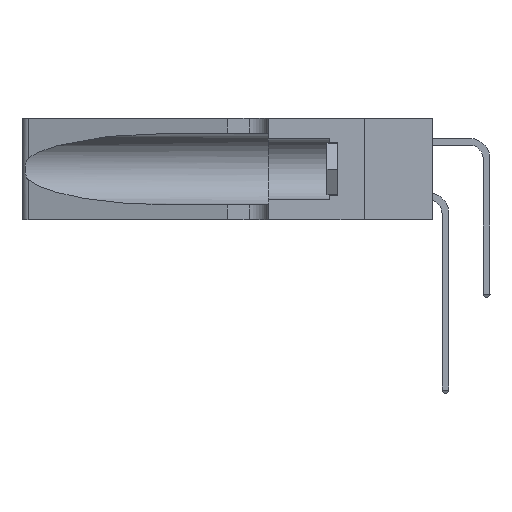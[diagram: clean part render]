
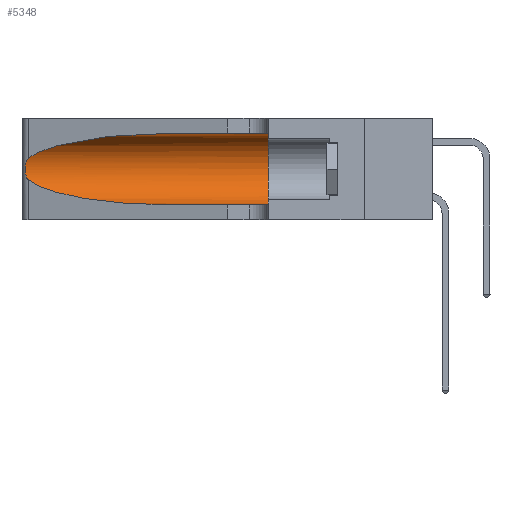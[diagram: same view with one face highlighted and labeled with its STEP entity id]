
A CAD part, left-side view. The second image highlights one B-rep face of the part: STEP entity #5348.
In plain terms, the highlighted cylindrical face has radius 3.308 mm (diameter 6.617 mm), a partial arc.
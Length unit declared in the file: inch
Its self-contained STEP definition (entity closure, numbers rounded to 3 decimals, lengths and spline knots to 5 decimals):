
#450 = B_SPLINE_CURVE_WITH_KNOTS ( 'NONE', 3,
 ( #13901, #22135, #18074, #5650, #20141, #7745, #22219, #9846, #24278, #11929, #26351, #13994, #1385, #16044 ),
 .UNSPECIFIED., .F., .F.,
 ( 4, 2, 2, 2, 2, 2, 4 ),
 ( 0., 0.00027, 0.00053, 0.00107, 0.0016, 0.00187, 0.00214 ),
 .UNSPECIFIED. ) ;
#459 = ORIENTED_EDGE ( 'NONE', *, *, #3956, .T. ) ;
#1385 = CARTESIAN_POINT ( 'NONE',  ( 0.25555, 1.22993, 0.14849 ) ) ;
#1475 =( BOUNDED_CURVE ( )  B_SPLINE_CURVE ( 3, ( #21719, #19643, #15539, #3058 ),
 .UNSPECIFIED., .F., .F. ) 
 B_SPLINE_CURVE_WITH_KNOTS ( ( 4, 4 ),
 ( 3.44316, 4.71239 ),
 .UNSPECIFIED. ) 
 CURVE ( )  GEOMETRIC_REPRESENTATION_ITEM ( )  RATIONAL_B_SPLINE_CURVE ( ( 1., 0.87, 0.87, 1. ) ) 
 REPRESENTATION_ITEM ( '' )  );
#1783 = LINE ( 'NONE', #19438, #17848 ) ;
#1936 = FACE_OUTER_BOUND ( 'NONE', #20420, .T. ) ;
#2734 = CARTESIAN_POINT ( 'NONE',  ( 0.1305, 0.35, 0.05475 ) ) ;
#3058 = CARTESIAN_POINT ( 'NONE',  ( 0.1305, 0.72297, 0.05475 ) ) ;
#3063 = VERTEX_POINT ( 'NONE', #4039 ) ;
#3956 = EDGE_CURVE ( 'NONE', #25879, #3063, #1475, .T. ) ;
#4039 = CARTESIAN_POINT ( 'NONE',  ( 0.1305, 0.72297, 0.05475 ) ) ;
#4221 = CARTESIAN_POINT ( 'NONE',  ( 0.2373, 1.15595, 0.28018 ) ) ;
#5104 = ORIENTED_EDGE ( 'NONE', *, *, #26479, .T. ) ;
#5348 = ADVANCED_FACE ( 'NONE', ( #1936 ), #12500, .F. ) ;
#5650 = CARTESIAN_POINT ( 'NONE',  ( 0.25787, 1.23484, 0.2124 ) ) ;
#6771 = ORIENTED_EDGE ( 'NONE', *, *, #18548, .F. ) ;
#6823 = LINE ( 'NONE', #25833, #17170 ) ;
#7297 = DIRECTION ( 'NONE',  ( 0., 1., 0. ) ) ;
#7745 = CARTESIAN_POINT ( 'NONE',  ( 0.26018, 1.23835, 0.19895 ) ) ;
#8367 = CARTESIAN_POINT ( 'NONE',  ( 0.1305, 0.72297, 0.31525 ) ) ;
#9005 = CARTESIAN_POINT ( 'NONE',  ( 0.1305, 0.35, 0.31525 ) ) ;
#9461 = CARTESIAN_POINT ( 'NONE',  ( 0.1305, 1.61858, 0.185 ) ) ;
#9760 = EDGE_CURVE ( 'NONE', #14841, #25879, #450, .T. ) ;
#9846 = CARTESIAN_POINT ( 'NONE',  ( 0.26075, 1.23896, 0.178 ) ) ;
#11261 = EDGE_CURVE ( 'NONE', #23803, #24800, #1783, .T. ) ;
#11929 = CARTESIAN_POINT ( 'NONE',  ( 0.25856, 1.23593, 0.16098 ) ) ;
#12500 = CYLINDRICAL_SURFACE ( 'NONE', #20437, 0.13025 ) ;
#13292 = DIRECTION ( 'NONE',  ( 0., -1., 0. ) ) ;
#13480 = DIRECTION ( 'NONE',  ( 0., -1., 0. ) ) ;
#13796 =( BOUNDED_CURVE ( )  B_SPLINE_CURVE ( 3, ( #8367, #20746, #4221, #18765 ),
 .UNSPECIFIED., .F., .F. ) 
 B_SPLINE_CURVE_WITH_KNOTS ( ( 4, 4 ),
 ( 1.5708, 2.84003 ),
 .UNSPECIFIED. ) 
 CURVE ( )  GEOMETRIC_REPRESENTATION_ITEM ( )  RATIONAL_B_SPLINE_CURVE ( ( 1., 0.87, 0.87, 1. ) ) 
 REPRESENTATION_ITEM ( '' )  );
#13901 = CARTESIAN_POINT ( 'NONE',  ( 0.25487, 1.22718, 0.22369 ) ) ;
#13994 = CARTESIAN_POINT ( 'NONE',  ( 0.25639, 1.23186, 0.15144 ) ) ;
#14841 = VERTEX_POINT ( 'NONE', #15242 ) ;
#15242 = CARTESIAN_POINT ( 'NONE',  ( 0.25487, 1.22718, 0.22369 ) ) ;
#15539 = CARTESIAN_POINT ( 'NONE',  ( 0.18966, 0.96281, 0.05475 ) ) ;
#16044 = CARTESIAN_POINT ( 'NONE',  ( 0.25487, 1.22718, 0.14631 ) ) ;
#17170 = VECTOR ( 'NONE', #13480, 39.37008 ) ;
#17848 = VECTOR ( 'NONE', #13292, 39.37008 ) ;
#18074 = CARTESIAN_POINT ( 'NONE',  ( 0.25639, 1.23184, 0.21858 ) ) ;
#18548 = EDGE_CURVE ( 'NONE', #24800, #24177, #18861, .T. ) ;
#18765 = CARTESIAN_POINT ( 'NONE',  ( 0.25487, 1.22718, 0.22369 ) ) ;
#18861 = CIRCLE ( 'NONE', #19857, 0.13025 ) ;
#19438 = CARTESIAN_POINT ( 'NONE',  ( 0.1305, 1.61858, 0.31525 ) ) ;
#19643 = CARTESIAN_POINT ( 'NONE',  ( 0.2373, 1.15595, 0.08982 ) ) ;
#19686 = CARTESIAN_POINT ( 'NONE',  ( 0.1305, 0.35, 0.185 ) ) ;
#19750 = DIRECTION ( 'NONE',  ( 0., 0., -1. ) ) ;
#19857 = AXIS2_PLACEMENT_3D ( 'NONE', #19686, #7297, #21771 ) ;
#20141 = CARTESIAN_POINT ( 'NONE',  ( 0.25854, 1.2359, 0.20912 ) ) ;
#20420 = EDGE_LOOP ( 'NONE', ( #5104, #22215, #459, #22430, #6771, #24650 ) ) ;
#20437 = AXIS2_PLACEMENT_3D ( 'NONE', #9461, #23882, #19750 ) ;
#20746 = CARTESIAN_POINT ( 'NONE',  ( 0.18966, 0.96281, 0.31525 ) ) ;
#21719 = CARTESIAN_POINT ( 'NONE',  ( 0.25487, 1.22718, 0.14631 ) ) ;
#21771 = DIRECTION ( 'NONE',  ( 0., 0., 1. ) ) ;
#22135 = CARTESIAN_POINT ( 'NONE',  ( 0.25555, 1.22994, 0.2215 ) ) ;
#22215 = ORIENTED_EDGE ( 'NONE', *, *, #9760, .T. ) ;
#22219 = CARTESIAN_POINT ( 'NONE',  ( 0.26075, 1.23896, 0.19203 ) ) ;
#22430 = ORIENTED_EDGE ( 'NONE', *, *, #25527, .T. ) ;
#22752 = CARTESIAN_POINT ( 'NONE',  ( 0.25487, 1.22718, 0.14631 ) ) ;
#23803 = VERTEX_POINT ( 'NONE', #24338 ) ;
#23882 = DIRECTION ( 'NONE',  ( 0., -1., 0. ) ) ;
#24177 = VERTEX_POINT ( 'NONE', #2734 ) ;
#24278 = CARTESIAN_POINT ( 'NONE',  ( 0.26017, 1.23833, 0.17102 ) ) ;
#24338 = CARTESIAN_POINT ( 'NONE',  ( 0.1305, 0.72297, 0.31525 ) ) ;
#24650 = ORIENTED_EDGE ( 'NONE', *, *, #11261, .F. ) ;
#24800 = VERTEX_POINT ( 'NONE', #9005 ) ;
#25527 = EDGE_CURVE ( 'NONE', #3063, #24177, #6823, .T. ) ;
#25833 = CARTESIAN_POINT ( 'NONE',  ( 0.1305, 1.61858, 0.05475 ) ) ;
#25879 = VERTEX_POINT ( 'NONE', #22752 ) ;
#26351 = CARTESIAN_POINT ( 'NONE',  ( 0.25789, 1.23486, 0.15765 ) ) ;
#26479 = EDGE_CURVE ( 'NONE', #23803, #14841, #13796, .T. ) ;
